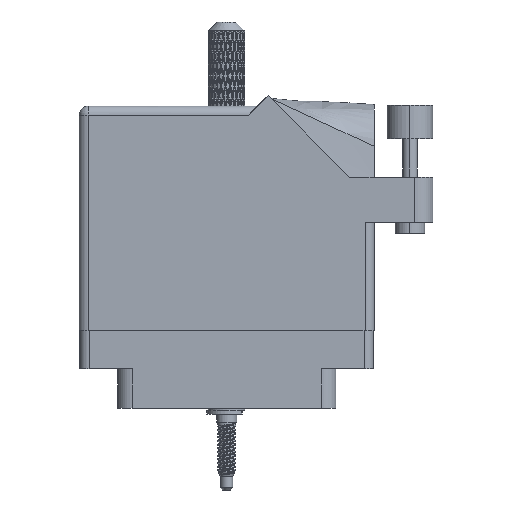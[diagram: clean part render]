
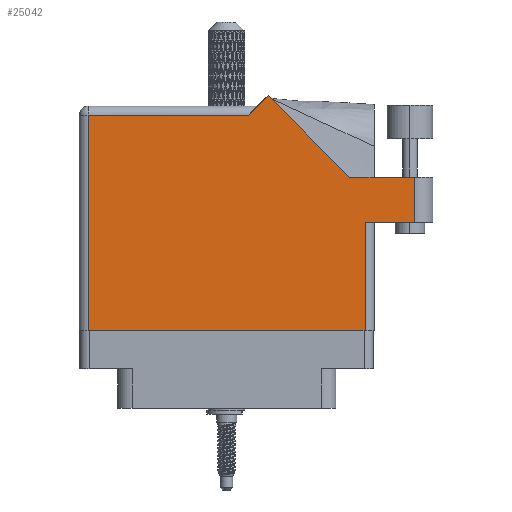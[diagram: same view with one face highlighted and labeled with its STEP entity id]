
A CAD part, front view. The second image highlights one B-rep face of the part: STEP entity #25042.
In plain terms, the highlighted face is planar.
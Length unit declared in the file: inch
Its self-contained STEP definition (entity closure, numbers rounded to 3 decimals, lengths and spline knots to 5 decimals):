
#3255 = CARTESIAN_POINT ( 'NONE',  ( 2.285, 1.044, 0. ) ) ;
#4733 = PLANE ( 'NONE',  #43014 ) ;
#6159 = DIRECTION ( 'NONE',  ( -0.707, -0.707, 0. ) ) ;
#7544 = ORIENTED_EDGE ( 'NONE', *, *, #76593, .T. ) ;
#10698 = EDGE_CURVE ( 'NONE', #50855, #31898, #54050, .T. ) ;
#11761 = DIRECTION ( 'NONE',  ( 0., 1., 0. ) ) ;
#13987 = EDGE_CURVE ( 'NONE', #99454, #41315, #53703, .T. ) ;
#14033 = CARTESIAN_POINT ( 'NONE',  ( 1.217, 1.53, 0. ) ) ;
#14072 = ORIENTED_EDGE ( 'NONE', *, *, #31529, .T. ) ;
#18080 = CARTESIAN_POINT ( 'NONE',  ( 1.84442, 1.044, 0. ) ) ;
#18940 = CARTESIAN_POINT ( 'NONE',  ( 2.285, 0.737, 0. ) ) ;
#19442 = LINE ( 'NONE', #27397, #57454 ) ;
#21173 = VERTEX_POINT ( 'NONE', #62082 ) ;
#21895 = FACE_OUTER_BOUND ( 'NONE', #60212, .T. ) ;
#22704 = ORIENTED_EDGE ( 'NONE', *, *, #74528, .T. ) ;
#23545 = VECTOR ( 'NONE', #6159, 39.37008 ) ;
#24216 = VERTEX_POINT ( 'NONE', #77516 ) ;
#24532 = VERTEX_POINT ( 'NONE', #99957 ) ;
#25042 = ADVANCED_FACE ( 'NONE', ( #21895 ), #4733, .F. ) ;
#26849 = DIRECTION ( 'NONE',  ( 1., 0., 0. ) ) ;
#27176 = CARTESIAN_POINT ( 'NONE',  ( 0.062, 0., 0. ) ) ;
#27268 = ORIENTED_EDGE ( 'NONE', *, *, #10698, .T. ) ;
#27397 = CARTESIAN_POINT ( 'NONE',  ( 1.948, 0.737, 0. ) ) ;
#27523 = DIRECTION ( 'NONE',  ( 0., -1., 0. ) ) ;
#27981 = CARTESIAN_POINT ( 'NONE',  ( 1.84442, 1.044, 0. ) ) ;
#31206 = VECTOR ( 'NONE', #27523, 39.37008 ) ;
#31529 = EDGE_CURVE ( 'NONE', #21173, #66091, #96560, .T. ) ;
#31898 = VERTEX_POINT ( 'NONE', #27981 ) ;
#32063 = ORIENTED_EDGE ( 'NONE', *, *, #35743, .T. ) ;
#35743 = EDGE_CURVE ( 'NONE', #24532, #24216, #45089, .T. ) ;
#35906 = DIRECTION ( 'NONE',  ( 0., 1., 0. ) ) ;
#37367 = DIRECTION ( 'NONE',  ( -1., 0., 0. ) ) ;
#38425 = CARTESIAN_POINT ( 'NONE',  ( 0., 1.468, 0. ) ) ;
#40278 = CARTESIAN_POINT ( 'NONE',  ( 0.062, 0., 0. ) ) ;
#41279 = VECTOR ( 'NONE', #35906, 39.37008 ) ;
#41315 = VERTEX_POINT ( 'NONE', #47857 ) ;
#41504 = ORIENTED_EDGE ( 'NONE', *, *, #13987, .T. ) ;
#43014 = AXIS2_PLACEMENT_3D ( 'NONE', #93841, #69510, #37367 ) ;
#43617 = ORIENTED_EDGE ( 'NONE', *, *, #69973, .T. ) ;
#45089 = LINE ( 'NONE', #14033, #23545 ) ;
#45763 = CARTESIAN_POINT ( 'NONE',  ( 2.41, 1.044, 0. ) ) ;
#46087 = VECTOR ( 'NONE', #82823, 39.37008 ) ;
#47857 = CARTESIAN_POINT ( 'NONE',  ( 1.948, 0., 0. ) ) ;
#48832 = LINE ( 'NONE', #27176, #31206 ) ;
#50855 = VERTEX_POINT ( 'NONE', #3255 ) ;
#51478 = LINE ( 'NONE', #38425, #94386 ) ;
#53703 = LINE ( 'NONE', #74726, #46087 ) ;
#54050 = LINE ( 'NONE', #45763, #101964 ) ;
#57454 = VECTOR ( 'NONE', #11761, 39.37008 ) ;
#58827 = VERTEX_POINT ( 'NONE', #68304 ) ;
#58965 = VECTOR ( 'NONE', #66224, 39.37008 ) ;
#60212 = EDGE_LOOP ( 'NONE', ( #14072, #83511, #27268, #22704, #32063, #67572, #43617, #41504, #7544 ) ) ;
#62082 = CARTESIAN_POINT ( 'NONE',  ( 1.948, 0.737, 0. ) ) ;
#66091 = VERTEX_POINT ( 'NONE', #18940 ) ;
#66224 = DIRECTION ( 'NONE',  ( -0.707, 0.707, 0. ) ) ;
#67572 = ORIENTED_EDGE ( 'NONE', *, *, #68261, .T. ) ;
#68261 = EDGE_CURVE ( 'NONE', #24216, #58827, #51478, .T. ) ;
#68304 = CARTESIAN_POINT ( 'NONE',  ( 0.062, 1.468, 0. ) ) ;
#69510 = DIRECTION ( 'NONE',  ( 0., 0., -1. ) ) ;
#69973 = EDGE_CURVE ( 'NONE', #58827, #99454, #48832, .T. ) ;
#70531 = EDGE_CURVE ( 'NONE', #66091, #50855, #95506, .T. ) ;
#74528 = EDGE_CURVE ( 'NONE', #31898, #24532, #90516, .T. ) ;
#74726 = CARTESIAN_POINT ( 'NONE',  ( 0., 0., 0. ) ) ;
#76593 = EDGE_CURVE ( 'NONE', #41315, #21173, #19442, .T. ) ;
#77516 = CARTESIAN_POINT ( 'NONE',  ( 1.155, 1.468, 0. ) ) ;
#82823 = DIRECTION ( 'NONE',  ( 1., 0., 0. ) ) ;
#83511 = ORIENTED_EDGE ( 'NONE', *, *, #70531, .T. ) ;
#85947 = DIRECTION ( 'NONE',  ( -1., 0., 0. ) ) ;
#90516 = LINE ( 'NONE', #18080, #58965 ) ;
#93841 = CARTESIAN_POINT ( 'NONE',  ( 0., 1.53, 0. ) ) ;
#94386 = VECTOR ( 'NONE', #94868, 39.37008 ) ;
#94868 = DIRECTION ( 'NONE',  ( -1., 0., 0. ) ) ;
#95506 = LINE ( 'NONE', #99037, #41279 ) ;
#96560 = LINE ( 'NONE', #99541, #99100 ) ;
#99037 = CARTESIAN_POINT ( 'NONE',  ( 2.285, 1.044, 0. ) ) ;
#99100 = VECTOR ( 'NONE', #26849, 39.37008 ) ;
#99454 = VERTEX_POINT ( 'NONE', #40278 ) ;
#99541 = CARTESIAN_POINT ( 'NONE',  ( 2.01, 0.737, 0. ) ) ;
#99957 = CARTESIAN_POINT ( 'NONE',  ( 1.28771, 1.60071, 0. ) ) ;
#101964 = VECTOR ( 'NONE', #85947, 39.37008 ) ;
